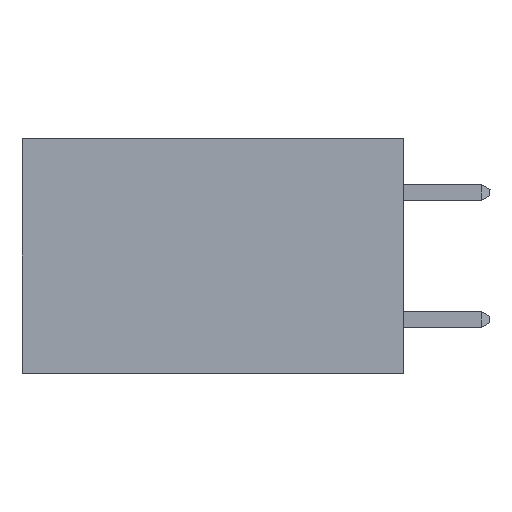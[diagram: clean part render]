
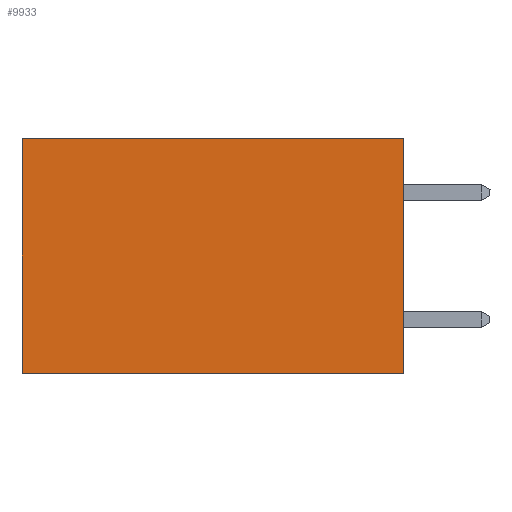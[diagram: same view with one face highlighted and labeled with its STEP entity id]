
A CAD part, left-side view. The second image highlights one B-rep face of the part: STEP entity #9933.
In plain terms, the highlighted planar face has unit normal (-1, 0, 0).
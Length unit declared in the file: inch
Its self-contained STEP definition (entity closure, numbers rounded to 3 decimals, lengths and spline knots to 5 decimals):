
#154 = VERTEX_POINT ( 'NONE', #7013 ) ;
#1805 = CARTESIAN_POINT ( 'NONE',  ( 0.2875, 0., 0. ) ) ;
#2346 = VERTEX_POINT ( 'NONE', #8115 ) ;
#2539 = CARTESIAN_POINT ( 'NONE',  ( 0.2875, 0., -0.37 ) ) ;
#2542 = DIRECTION ( 'NONE',  ( 0., 0., -1. ) ) ;
#3007 = EDGE_CURVE ( 'NONE', #154, #2346, #13944, .T. ) ;
#3700 = DIRECTION ( 'NONE',  ( 0., 1., 0. ) ) ;
#4416 = DIRECTION ( 'NONE',  ( 0., 0., -1. ) ) ;
#5936 = ORIENTED_EDGE ( 'NONE', *, *, #8387, .F. ) ;
#7013 = CARTESIAN_POINT ( 'NONE',  ( 0.2875, 0., 0. ) ) ;
#7493 = PLANE ( 'NONE',  #16179 ) ;
#7936 = EDGE_LOOP ( 'NONE', ( #22518, #13338, #5936, #20443 ) ) ;
#8115 = CARTESIAN_POINT ( 'NONE',  ( 0.2875, 0.6, 0. ) ) ;
#8387 = EDGE_CURVE ( 'NONE', #154, #8544, #12901, .T. ) ;
#8544 = VERTEX_POINT ( 'NONE', #2539 ) ;
#8772 = DIRECTION ( 'NONE',  ( 0., 1., 0. ) ) ;
#9102 = VECTOR ( 'NONE', #8772, 39.37008 ) ;
#9933 = ADVANCED_FACE ( 'NONE', ( #21167 ), #7493, .F. ) ;
#9935 = CARTESIAN_POINT ( 'NONE',  ( 0.2875, 0., 0. ) ) ;
#11939 = CARTESIAN_POINT ( 'NONE',  ( 0.2875, 0.6, 0. ) ) ;
#12336 = VECTOR ( 'NONE', #4416, 39.37008 ) ;
#12901 = LINE ( 'NONE', #9935, #12336 ) ;
#13338 = ORIENTED_EDGE ( 'NONE', *, *, #23481, .F. ) ;
#13944 = LINE ( 'NONE', #1805, #9102 ) ;
#14420 = LINE ( 'NONE', #11939, #15296 ) ;
#14570 = CARTESIAN_POINT ( 'NONE',  ( 0.2875, 0., -0.37 ) ) ;
#14572 = DIRECTION ( 'NONE',  ( 0., 0., -1. ) ) ;
#15296 = VECTOR ( 'NONE', #2542, 39.37008 ) ;
#16179 = AXIS2_PLACEMENT_3D ( 'NONE', #21936, #22000, #14572 ) ;
#19842 = LINE ( 'NONE', #14570, #21251 ) ;
#20443 = ORIENTED_EDGE ( 'NONE', *, *, #3007, .T. ) ;
#20597 = CARTESIAN_POINT ( 'NONE',  ( 0.2875, 0.6, -0.37 ) ) ;
#20838 = VERTEX_POINT ( 'NONE', #20597 ) ;
#21167 = FACE_OUTER_BOUND ( 'NONE', #7936, .T. ) ;
#21251 = VECTOR ( 'NONE', #3700, 39.37008 ) ;
#21936 = CARTESIAN_POINT ( 'NONE',  ( 0.2875, 0., 0. ) ) ;
#22000 = DIRECTION ( 'NONE',  ( 1., 0., 0. ) ) ;
#22518 = ORIENTED_EDGE ( 'NONE', *, *, #22527, .T. ) ;
#22527 = EDGE_CURVE ( 'NONE', #2346, #20838, #14420, .T. ) ;
#23481 = EDGE_CURVE ( 'NONE', #8544, #20838, #19842, .T. ) ;
